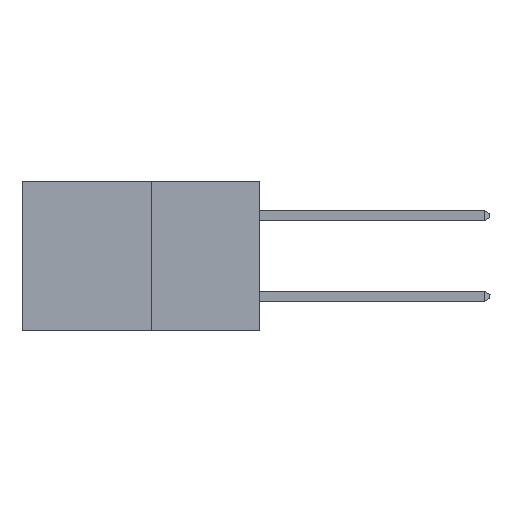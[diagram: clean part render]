
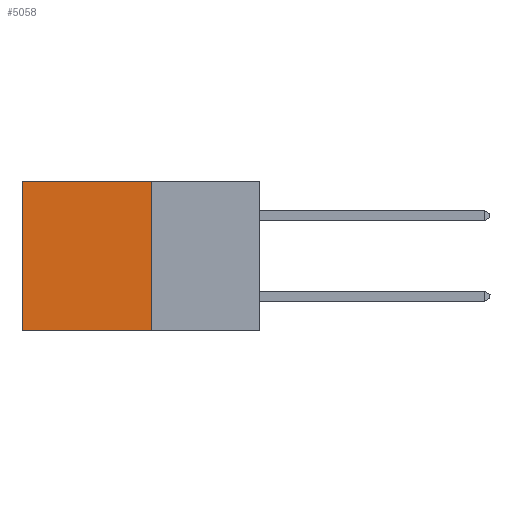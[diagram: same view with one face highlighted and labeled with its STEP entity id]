
A CAD part, left-side view. The second image highlights one B-rep face of the part: STEP entity #5058.
In plain terms, the highlighted planar face has unit normal (-1, 0, 0).
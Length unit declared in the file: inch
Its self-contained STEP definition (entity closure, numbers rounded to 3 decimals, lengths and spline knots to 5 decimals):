
#459 = CARTESIAN_POINT ( 'NONE',  ( 0.277, 0.59, 0. ) ) ;
#516 = VECTOR ( 'NONE', #9862, 39.37008 ) ;
#611 = DIRECTION ( 'NONE',  ( 1., 0., 0. ) ) ;
#969 = ORIENTED_EDGE ( 'NONE', *, *, #9988, .T. ) ;
#998 = ORIENTED_EDGE ( 'NONE', *, *, #2199, .F. ) ;
#1072 = ORIENTED_EDGE ( 'NONE', *, *, #1671, .F. ) ;
#1106 = ORIENTED_EDGE ( 'NONE', *, *, #5197, .T. ) ;
#1671 = EDGE_CURVE ( 'NONE', #3375, #4078, #4345, .T. ) ;
#1860 = VERTEX_POINT ( 'NONE', #3175 ) ;
#2057 = VECTOR ( 'NONE', #6331, 39.37008 ) ;
#2199 = EDGE_CURVE ( 'NONE', #4078, #1860, #5240, .T. ) ;
#3096 = AXIS2_PLACEMENT_3D ( 'NONE', #8792, #611, #6626 ) ;
#3098 = LINE ( 'NONE', #6006, #9281 ) ;
#3175 = CARTESIAN_POINT ( 'NONE',  ( 0.277, 0.59, -0.37 ) ) ;
#3302 = PLANE ( 'NONE',  #3096 ) ;
#3375 = VERTEX_POINT ( 'NONE', #7523 ) ;
#4078 = VERTEX_POINT ( 'NONE', #4847 ) ;
#4345 = LINE ( 'NONE', #6155, #2057 ) ;
#4712 = FACE_OUTER_BOUND ( 'NONE', #6696, .T. ) ;
#4847 = CARTESIAN_POINT ( 'NONE',  ( 0.277, 0.27, -0.37 ) ) ;
#5058 = ADVANCED_FACE ( 'NONE', ( #4712 ), #3302, .F. ) ;
#5197 = EDGE_CURVE ( 'NONE', #3375, #8507, #3098, .T. ) ;
#5240 = LINE ( 'NONE', #9984, #516 ) ;
#5394 = DIRECTION ( 'NONE',  ( 0., 0., -1. ) ) ;
#6006 = CARTESIAN_POINT ( 'NONE',  ( 0.277, 0.27, 0. ) ) ;
#6155 = CARTESIAN_POINT ( 'NONE',  ( 0.277, 0.27, -0.37 ) ) ;
#6331 = DIRECTION ( 'NONE',  ( 0., 0., -1. ) ) ;
#6626 = DIRECTION ( 'NONE',  ( 0., 0., -1. ) ) ;
#6696 = EDGE_LOOP ( 'NONE', ( #969, #998, #1072, #1106 ) ) ;
#6772 = LINE ( 'NONE', #7674, #8716 ) ;
#7523 = CARTESIAN_POINT ( 'NONE',  ( 0.277, 0.27, 0. ) ) ;
#7674 = CARTESIAN_POINT ( 'NONE',  ( 0.277, 0.59, -0.37 ) ) ;
#8507 = VERTEX_POINT ( 'NONE', #459 ) ;
#8716 = VECTOR ( 'NONE', #5394, 39.37008 ) ;
#8792 = CARTESIAN_POINT ( 'NONE',  ( 0.277, 0.27, -0.37 ) ) ;
#9281 = VECTOR ( 'NONE', #10331, 39.37008 ) ;
#9862 = DIRECTION ( 'NONE',  ( 0., 1., 0. ) ) ;
#9984 = CARTESIAN_POINT ( 'NONE',  ( 0.277, 0.27, -0.37 ) ) ;
#9988 = EDGE_CURVE ( 'NONE', #8507, #1860, #6772, .T. ) ;
#10331 = DIRECTION ( 'NONE',  ( 0., 1., 0. ) ) ;
